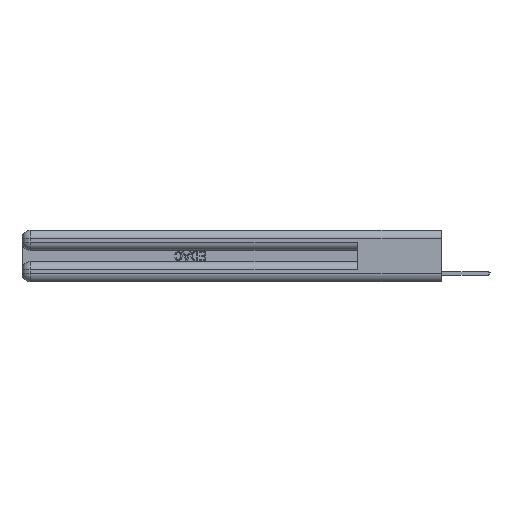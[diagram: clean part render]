
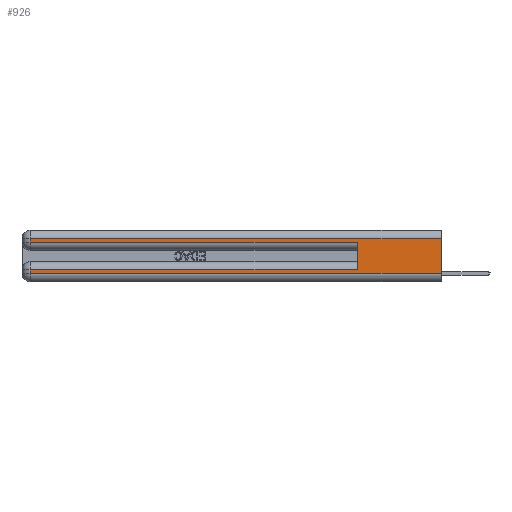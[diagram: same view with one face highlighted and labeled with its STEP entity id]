
A CAD part, left-side view. The second image highlights one B-rep face of the part: STEP entity #926.
In plain terms, the highlighted planar face has unit normal (-1, 0, 0).
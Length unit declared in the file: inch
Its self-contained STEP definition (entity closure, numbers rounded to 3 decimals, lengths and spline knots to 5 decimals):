
#663 = ORIENTED_EDGE ( 'NONE', *, *, #31115, .T. ) ;
#926 = ADVANCED_FACE ( 'NONE', ( #22587 ), #32670, .F. ) ;
#1540 = ORIENTED_EDGE ( 'NONE', *, *, #8575, .T. ) ;
#1943 = CARTESIAN_POINT ( 'NONE',  ( 0., 0.6, 0.085 ) ) ;
#2426 = CARTESIAN_POINT ( 'NONE',  ( 0., 2.94, 0.285 ) ) ;
#3756 = VECTOR ( 'NONE', #17433, 39.37008 ) ;
#3889 = EDGE_CURVE ( 'NONE', #5021, #29813, #30187, .T. ) ;
#3960 = VECTOR ( 'NONE', #13385, 39.37008 ) ;
#3994 = CARTESIAN_POINT ( 'NONE',  ( 0., 0., 0.37 ) ) ;
#4475 = DIRECTION ( 'NONE',  ( 0., 0., -1. ) ) ;
#5021 = VERTEX_POINT ( 'NONE', #14757 ) ;
#5974 = VERTEX_POINT ( 'NONE', #1943 ) ;
#6416 = LINE ( 'NONE', #17004, #8978 ) ;
#6852 = EDGE_LOOP ( 'NONE', ( #21374, #1540, #29002, #32723, #32444, #30736, #663, #24251 ) ) ;
#7183 = CARTESIAN_POINT ( 'NONE',  ( 0., 0., 0.31 ) ) ;
#7191 = CARTESIAN_POINT ( 'NONE',  ( 0., 0., 0.06 ) ) ;
#7875 = CARTESIAN_POINT ( 'NONE',  ( 0., 2.94, 0.37 ) ) ;
#8218 = VECTOR ( 'NONE', #28870, 39.37008 ) ;
#8341 = LINE ( 'NONE', #14863, #16754 ) ;
#8575 = EDGE_CURVE ( 'NONE', #12138, #13700, #30178, .T. ) ;
#8715 = CARTESIAN_POINT ( 'NONE',  ( 0., 2.94, 0.37 ) ) ;
#8978 = VECTOR ( 'NONE', #26716, 39.37008 ) ;
#9603 = AXIS2_PLACEMENT_3D ( 'NONE', #3994, #16928, #32350 ) ;
#11230 = DIRECTION ( 'NONE',  ( 0., 0., -1. ) ) ;
#12138 = VERTEX_POINT ( 'NONE', #15135 ) ;
#13011 = EDGE_CURVE ( 'NONE', #22294, #28565, #28286, .T. ) ;
#13385 = DIRECTION ( 'NONE',  ( 0., 1., 0. ) ) ;
#13481 = CARTESIAN_POINT ( 'NONE',  ( 0., 2.94, 0.085 ) ) ;
#13501 = CARTESIAN_POINT ( 'NONE',  ( 0., 0.6, 0.285 ) ) ;
#13700 = VERTEX_POINT ( 'NONE', #15634 ) ;
#14160 = EDGE_CURVE ( 'NONE', #13700, #22294, #30890, .T. ) ;
#14479 = EDGE_CURVE ( 'NONE', #5974, #15449, #25477, .T. ) ;
#14757 = CARTESIAN_POINT ( 'NONE',  ( 0., 2.94, 0.06 ) ) ;
#14863 = CARTESIAN_POINT ( 'NONE',  ( 0., 0., 0.37 ) ) ;
#15071 = EDGE_CURVE ( 'NONE', #5974, #28565, #6416, .T. ) ;
#15135 = CARTESIAN_POINT ( 'NONE',  ( 0., 0., 0.31 ) ) ;
#15449 = VERTEX_POINT ( 'NONE', #13481 ) ;
#15634 = CARTESIAN_POINT ( 'NONE',  ( 0., 2.94, 0.31 ) ) ;
#15725 = CARTESIAN_POINT ( 'NONE',  ( 0., 0., 0.085 ) ) ;
#16754 = VECTOR ( 'NONE', #4475, 39.37008 ) ;
#16770 = VECTOR ( 'NONE', #11230, 39.37008 ) ;
#16928 = DIRECTION ( 'NONE',  ( 1., 0., 0. ) ) ;
#17004 = CARTESIAN_POINT ( 'NONE',  ( 0., 0.6, 0.145 ) ) ;
#17433 = DIRECTION ( 'NONE',  ( 0., 1., 0. ) ) ;
#17446 = DIRECTION ( 'NONE',  ( 0., -1., 0. ) ) ;
#18373 = CARTESIAN_POINT ( 'NONE',  ( 0., 0., 0.06 ) ) ;
#20409 = EDGE_CURVE ( 'NONE', #12138, #29813, #8341, .T. ) ;
#21057 = VECTOR ( 'NONE', #17446, 39.37008 ) ;
#21374 = ORIENTED_EDGE ( 'NONE', *, *, #20409, .F. ) ;
#22136 = CARTESIAN_POINT ( 'NONE',  ( 0., 0., 0.285 ) ) ;
#22293 = VECTOR ( 'NONE', #29695, 39.37008 ) ;
#22294 = VERTEX_POINT ( 'NONE', #2426 ) ;
#22587 = FACE_OUTER_BOUND ( 'NONE', #6852, .T. ) ;
#24251 = ORIENTED_EDGE ( 'NONE', *, *, #3889, .T. ) ;
#25477 = LINE ( 'NONE', #15725, #3960 ) ;
#26332 = LINE ( 'NONE', #8715, #8218 ) ;
#26716 = DIRECTION ( 'NONE',  ( 0., 0., 1. ) ) ;
#28286 = LINE ( 'NONE', #22136, #22293 ) ;
#28565 = VERTEX_POINT ( 'NONE', #13501 ) ;
#28870 = DIRECTION ( 'NONE',  ( 0., 0., -1. ) ) ;
#29002 = ORIENTED_EDGE ( 'NONE', *, *, #14160, .T. ) ;
#29695 = DIRECTION ( 'NONE',  ( 0., -1., 0. ) ) ;
#29813 = VERTEX_POINT ( 'NONE', #18373 ) ;
#30178 = LINE ( 'NONE', #7183, #3756 ) ;
#30187 = LINE ( 'NONE', #7191, #21057 ) ;
#30736 = ORIENTED_EDGE ( 'NONE', *, *, #14479, .T. ) ;
#30890 = LINE ( 'NONE', #7875, #16770 ) ;
#31115 = EDGE_CURVE ( 'NONE', #15449, #5021, #26332, .T. ) ;
#32350 = DIRECTION ( 'NONE',  ( 0., 0., -1. ) ) ;
#32444 = ORIENTED_EDGE ( 'NONE', *, *, #15071, .F. ) ;
#32670 = PLANE ( 'NONE',  #9603 ) ;
#32723 = ORIENTED_EDGE ( 'NONE', *, *, #13011, .T. ) ;
